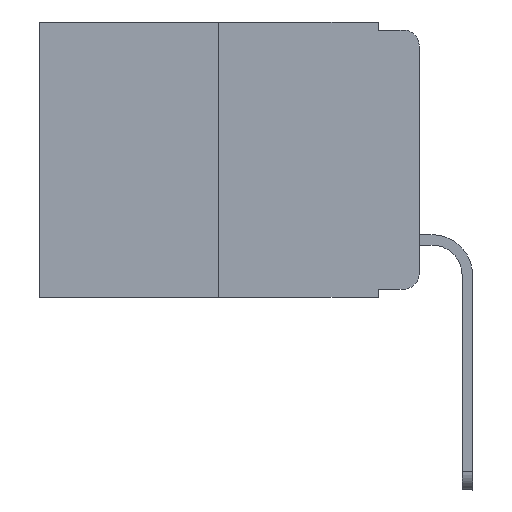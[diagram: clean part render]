
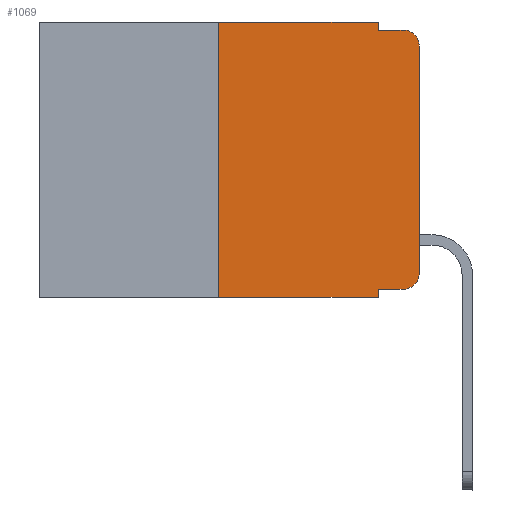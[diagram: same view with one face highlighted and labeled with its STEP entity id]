
A CAD part, left-side view. The second image highlights one B-rep face of the part: STEP entity #1069.
In plain terms, the highlighted planar face has unit normal (-1, 0, 0).
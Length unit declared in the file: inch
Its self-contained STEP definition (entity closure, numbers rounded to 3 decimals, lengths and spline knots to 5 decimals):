
#460 = CIRCLE ( 'NONE', #2861, 0.02 ) ;
#501 = AXIS2_PLACEMENT_3D ( 'NONE', #9447, #24618, #9313 ) ;
#555 = CARTESIAN_POINT ( 'NONE',  ( 0., 0.02, -0.01 ) ) ;
#1069 = ADVANCED_FACE ( 'NONE', ( #1808 ), #17330, .F. ) ;
#1600 = CARTESIAN_POINT ( 'NONE',  ( 0., 0.051, 0. ) ) ;
#1808 = FACE_OUTER_BOUND ( 'NONE', #6524, .T. ) ;
#1844 = LINE ( 'NONE', #18862, #10424 ) ;
#1985 = VERTEX_POINT ( 'NONE', #17155 ) ;
#2154 = ORIENTED_EDGE ( 'NONE', *, *, #15623, .F. ) ;
#2679 = EDGE_CURVE ( 'NONE', #24607, #20402, #14475, .T. ) ;
#2861 = AXIS2_PLACEMENT_3D ( 'NONE', #13533, #19691, #9804 ) ;
#2917 = DIRECTION ( 'NONE',  ( 0., 0., -1. ) ) ;
#3163 = DIRECTION ( 'NONE',  ( -1., 0., 0. ) ) ;
#3363 = CARTESIAN_POINT ( 'NONE',  ( 0., 0.02, -0.333 ) ) ;
#3681 = CARTESIAN_POINT ( 'NONE',  ( 0., 0.051, -0.343 ) ) ;
#3783 = EDGE_CURVE ( 'NONE', #4855, #1985, #17370, .T. ) ;
#4076 = ORIENTED_EDGE ( 'NONE', *, *, #7398, .F. ) ;
#4083 = CARTESIAN_POINT ( 'NONE',  ( 0., 0., -0.313 ) ) ;
#4431 = ORIENTED_EDGE ( 'NONE', *, *, #22165, .F. ) ;
#4573 = LINE ( 'NONE', #18333, #8568 ) ;
#4855 = VERTEX_POINT ( 'NONE', #1600 ) ;
#5199 = LINE ( 'NONE', #12828, #16011 ) ;
#5445 = VERTEX_POINT ( 'NONE', #555 ) ;
#6493 = EDGE_CURVE ( 'NONE', #19625, #4855, #5199, .T. ) ;
#6524 = EDGE_LOOP ( 'NONE', ( #10513, #7462, #2154, #7485, #22049, #4076, #21648, #4431, #8617, #8393 ) ) ;
#6584 = CARTESIAN_POINT ( 'NONE',  ( 0., 0.25, 0. ) ) ;
#7147 = EDGE_CURVE ( 'NONE', #21962, #5445, #460, .T. ) ;
#7196 = EDGE_CURVE ( 'NONE', #12484, #24607, #1844, .T. ) ;
#7398 = EDGE_CURVE ( 'NONE', #9662, #19625, #15855, .T. ) ;
#7462 = ORIENTED_EDGE ( 'NONE', *, *, #7147, .T. ) ;
#7485 = ORIENTED_EDGE ( 'NONE', *, *, #3783, .F. ) ;
#8349 = DIRECTION ( 'NONE',  ( 0., 0., 1. ) ) ;
#8393 = ORIENTED_EDGE ( 'NONE', *, *, #2679, .T. ) ;
#8568 = VECTOR ( 'NONE', #8704, 39.37008 ) ;
#8617 = ORIENTED_EDGE ( 'NONE', *, *, #7196, .T. ) ;
#8704 = DIRECTION ( 'NONE',  ( 0., -1., 0. ) ) ;
#9313 = DIRECTION ( 'NONE',  ( 0., 0., -1. ) ) ;
#9447 = CARTESIAN_POINT ( 'NONE',  ( 0., 0.473, 0. ) ) ;
#9662 = VERTEX_POINT ( 'NONE', #10768 ) ;
#9804 = DIRECTION ( 'NONE',  ( 0., 0., -1. ) ) ;
#10424 = VECTOR ( 'NONE', #13099, 39.37008 ) ;
#10513 = ORIENTED_EDGE ( 'NONE', *, *, #16575, .T. ) ;
#10768 = CARTESIAN_POINT ( 'NONE',  ( 0., 0.25, -0.343 ) ) ;
#10974 = CARTESIAN_POINT ( 'NONE',  ( 0., 0., 0. ) ) ;
#11283 = DIRECTION ( 'NONE',  ( 0., -1., 0. ) ) ;
#12243 = VECTOR ( 'NONE', #11283, 39.37008 ) ;
#12429 = CARTESIAN_POINT ( 'NONE',  ( 0., 0.02, -0.313 ) ) ;
#12484 = VERTEX_POINT ( 'NONE', #13720 ) ;
#12828 = CARTESIAN_POINT ( 'NONE',  ( 0., 0.473, 0. ) ) ;
#13099 = DIRECTION ( 'NONE',  ( 0., -1., 0. ) ) ;
#13268 = CARTESIAN_POINT ( 'NONE',  ( 0., 0.473, -0.343 ) ) ;
#13271 = AXIS2_PLACEMENT_3D ( 'NONE', #12429, #3163, #2917 ) ;
#13533 = CARTESIAN_POINT ( 'NONE',  ( 0., 0.02, -0.03 ) ) ;
#13720 = CARTESIAN_POINT ( 'NONE',  ( 0., 0.051, -0.333 ) ) ;
#14475 = CIRCLE ( 'NONE', #13271, 0.02 ) ;
#14590 = VECTOR ( 'NONE', #18849, 39.37008 ) ;
#15623 = EDGE_CURVE ( 'NONE', #1985, #5445, #4573, .T. ) ;
#15824 = LINE ( 'NONE', #23741, #22880 ) ;
#15855 = LINE ( 'NONE', #6584, #18821 ) ;
#15976 = DIRECTION ( 'NONE',  ( 0., 0., -1. ) ) ;
#16011 = VECTOR ( 'NONE', #20499, 39.37008 ) ;
#16575 = EDGE_CURVE ( 'NONE', #20402, #21962, #24769, .T. ) ;
#17088 = CARTESIAN_POINT ( 'NONE',  ( 0., 0.25, 0. ) ) ;
#17155 = CARTESIAN_POINT ( 'NONE',  ( 0., 0.051, -0.01 ) ) ;
#17330 = PLANE ( 'NONE',  #501 ) ;
#17370 = LINE ( 'NONE', #23275, #24419 ) ;
#17381 = EDGE_CURVE ( 'NONE', #9662, #22035, #18788, .T. ) ;
#18333 = CARTESIAN_POINT ( 'NONE',  ( 0., 0.051, -0.01 ) ) ;
#18788 = LINE ( 'NONE', #13268, #12243 ) ;
#18821 = VECTOR ( 'NONE', #8349, 39.37008 ) ;
#18849 = DIRECTION ( 'NONE',  ( 0., 0., 1. ) ) ;
#18862 = CARTESIAN_POINT ( 'NONE',  ( 0., 0.051, -0.333 ) ) ;
#19625 = VERTEX_POINT ( 'NONE', #17088 ) ;
#19691 = DIRECTION ( 'NONE',  ( -1., 0., 0. ) ) ;
#20402 = VERTEX_POINT ( 'NONE', #4083 ) ;
#20499 = DIRECTION ( 'NONE',  ( 0., -1., 0. ) ) ;
#21648 = ORIENTED_EDGE ( 'NONE', *, *, #17381, .T. ) ;
#21962 = VERTEX_POINT ( 'NONE', #24138 ) ;
#22035 = VERTEX_POINT ( 'NONE', #3681 ) ;
#22049 = ORIENTED_EDGE ( 'NONE', *, *, #6493, .F. ) ;
#22165 = EDGE_CURVE ( 'NONE', #12484, #22035, #15824, .T. ) ;
#22880 = VECTOR ( 'NONE', #23616, 39.37008 ) ;
#23275 = CARTESIAN_POINT ( 'NONE',  ( 0., 0.051, 0. ) ) ;
#23616 = DIRECTION ( 'NONE',  ( 0., 0., -1. ) ) ;
#23741 = CARTESIAN_POINT ( 'NONE',  ( 0., 0.051, 0. ) ) ;
#24138 = CARTESIAN_POINT ( 'NONE',  ( 0., 0., -0.03 ) ) ;
#24419 = VECTOR ( 'NONE', #15976, 39.37008 ) ;
#24607 = VERTEX_POINT ( 'NONE', #3363 ) ;
#24618 = DIRECTION ( 'NONE',  ( 1., 0., 0. ) ) ;
#24769 = LINE ( 'NONE', #10974, #14590 ) ;
